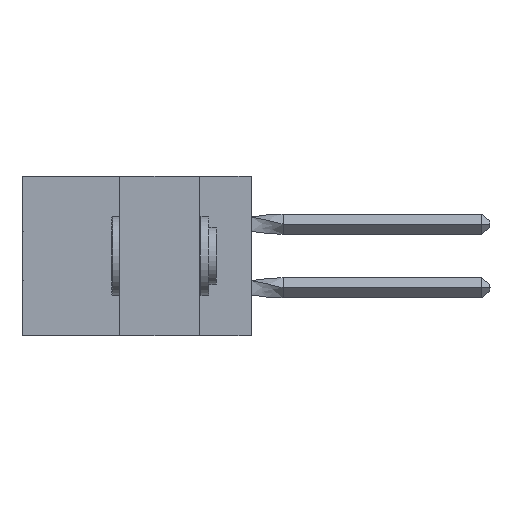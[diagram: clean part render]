
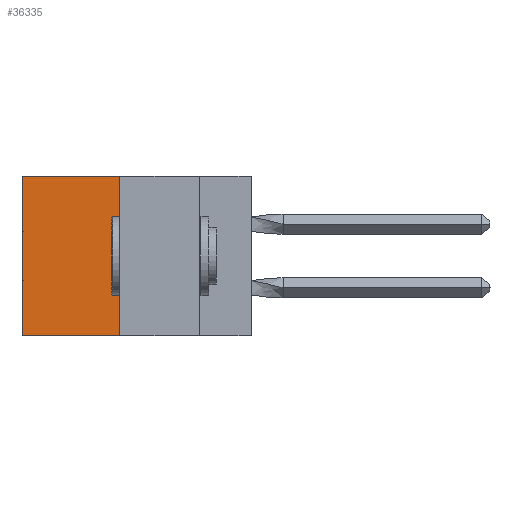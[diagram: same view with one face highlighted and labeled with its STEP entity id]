
A CAD part, left-side view. The second image highlights one B-rep face of the part: STEP entity #36335.
In plain terms, the highlighted planar face has unit normal (-1, 0, 0).
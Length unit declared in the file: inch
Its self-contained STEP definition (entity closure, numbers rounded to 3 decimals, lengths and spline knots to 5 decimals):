
#4115 = LINE ( 'NONE', #32915, #22826 ) ;
#4223 = VERTEX_POINT ( 'NONE', #27314 ) ;
#5371 = CARTESIAN_POINT ( 'NONE',  ( 0.305, 0.413, -0.5 ) ) ;
#5427 = VECTOR ( 'NONE', #12322, 39.37008 ) ;
#8463 = CARTESIAN_POINT ( 'NONE',  ( 0.305, 0.413, -0.5 ) ) ;
#10477 = LINE ( 'NONE', #44895, #5427 ) ;
#10797 = DIRECTION ( 'NONE',  ( 0., 0., -1. ) ) ;
#11002 = CARTESIAN_POINT ( 'NONE',  ( 0.305, 0.72, 0. ) ) ;
#12322 = DIRECTION ( 'NONE',  ( 0., 1., 0. ) ) ;
#13239 = DIRECTION ( 'NONE',  ( 1., 0., 0. ) ) ;
#13373 = LINE ( 'NONE', #25839, #41218 ) ;
#13572 = CARTESIAN_POINT ( 'NONE',  ( 0.305, 0.413, -0.5 ) ) ;
#14100 = EDGE_LOOP ( 'NONE', ( #15257, #15359, #24429, #38574 ) ) ;
#14647 = DIRECTION ( 'NONE',  ( 0., 0., -1. ) ) ;
#15257 = ORIENTED_EDGE ( 'NONE', *, *, #43909, .T. ) ;
#15359 = ORIENTED_EDGE ( 'NONE', *, *, #16031, .F. ) ;
#15922 = PLANE ( 'NONE',  #40476 ) ;
#16031 = EDGE_CURVE ( 'NONE', #37144, #4223, #17775, .T. ) ;
#17775 = LINE ( 'NONE', #8463, #32038 ) ;
#20123 = EDGE_CURVE ( 'NONE', #36957, #39492, #10477, .T. ) ;
#22826 = VECTOR ( 'NONE', #14647, 39.37008 ) ;
#24429 = ORIENTED_EDGE ( 'NONE', *, *, #27454, .F. ) ;
#25839 = CARTESIAN_POINT ( 'NONE',  ( 0.305, 0.413, -0.5 ) ) ;
#27314 = CARTESIAN_POINT ( 'NONE',  ( 0.305, 0.72, -0.5 ) ) ;
#27454 = EDGE_CURVE ( 'NONE', #36957, #37144, #13373, .T. ) ;
#31213 = DIRECTION ( 'NONE',  ( 0., 0., -1. ) ) ;
#32038 = VECTOR ( 'NONE', #41281, 39.37008 ) ;
#32915 = CARTESIAN_POINT ( 'NONE',  ( 0.305, 0.72, -0.5 ) ) ;
#36335 = ADVANCED_FACE ( 'NONE', ( #41132 ), #15922, .F. ) ;
#36957 = VERTEX_POINT ( 'NONE', #46652 ) ;
#37144 = VERTEX_POINT ( 'NONE', #13572 ) ;
#38574 = ORIENTED_EDGE ( 'NONE', *, *, #20123, .T. ) ;
#39492 = VERTEX_POINT ( 'NONE', #11002 ) ;
#40476 = AXIS2_PLACEMENT_3D ( 'NONE', #5371, #13239, #31213 ) ;
#41132 = FACE_OUTER_BOUND ( 'NONE', #14100, .T. ) ;
#41218 = VECTOR ( 'NONE', #10797, 39.37008 ) ;
#41281 = DIRECTION ( 'NONE',  ( 0., 1., 0. ) ) ;
#43909 = EDGE_CURVE ( 'NONE', #39492, #4223, #4115, .T. ) ;
#44895 = CARTESIAN_POINT ( 'NONE',  ( 0.305, 0.413, 0. ) ) ;
#46652 = CARTESIAN_POINT ( 'NONE',  ( 0.305, 0.413, 0. ) ) ;
